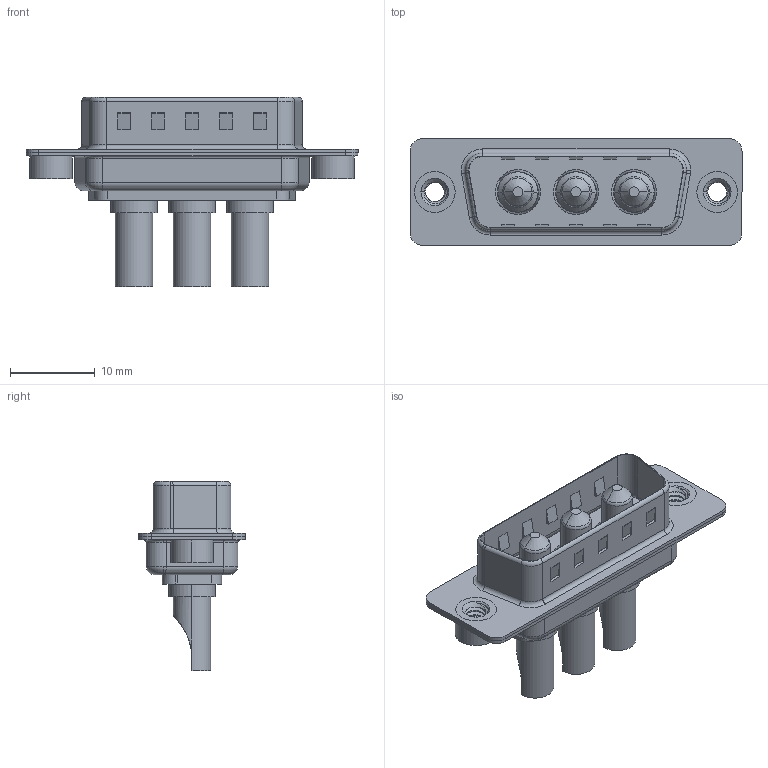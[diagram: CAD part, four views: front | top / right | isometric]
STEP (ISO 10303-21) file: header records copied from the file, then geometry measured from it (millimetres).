
FILE_DESCRIPTION (( 'STEP AP203' ), '1' );
FILE_NAME ('627-3W3-222-3T2.STEP', '2019-05-24T13:00:42', ( '' ), ( '' ), 'SwSTEP 2.0', 'SolidWorks 2016', '' );
FILE_SCHEMA (( 'CONFIG_CONTROL_DESIGN' ));
Length unit declared in the file: millimetre
Products named in the file (6): 627Combo Housing_3W3; 627Combo Shell Rear_15 Contacts; 627Combo Shell Front_15 Contacts; 627Combo Threaded Rivet_2; Power Pin_30A SC; 627-3W3-222-3T2
Assembly tree (8 placements, depth 2):
  627-3W3-222-3T2
    627Combo Housing_3W3
    627Combo Shell Rear_15 Contacts
    627Combo Shell Front_15 Contacts
    627Combo Threaded Rivet_2  x2
    Power Pin_30A SC  x3
Bounding box: 39.15 x 12.6 x 22.3 mm (x, y, z)
Volume: 2121.3 mm3; surface area: 5029.3 mm2
Topology: 11 solids, 11 shells, 478 faces, 1163 edges, 721 vertices
Faces by surface type: cylinder 199, plane 178, torus 56, cone 33, bspline 12
Entity records: 13022 total; most frequent: CARTESIAN_POINT 3479, DIRECTION 1928, ORIENTED_EDGE 1796, EDGE_CURVE 898, AXIS2_PLACEMENT_3D 716, VERTEX_POINT 563, VECTOR 496, LINE 496
